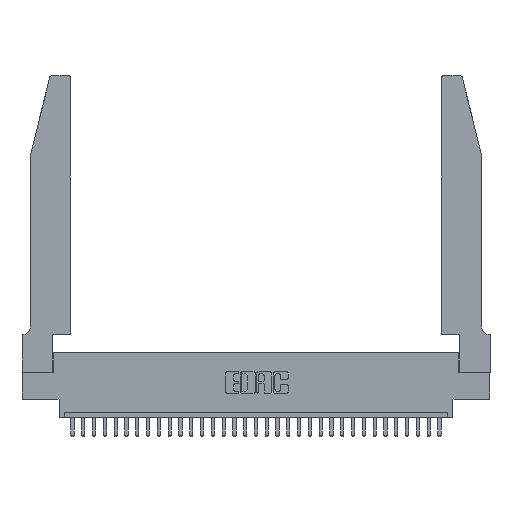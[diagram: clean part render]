
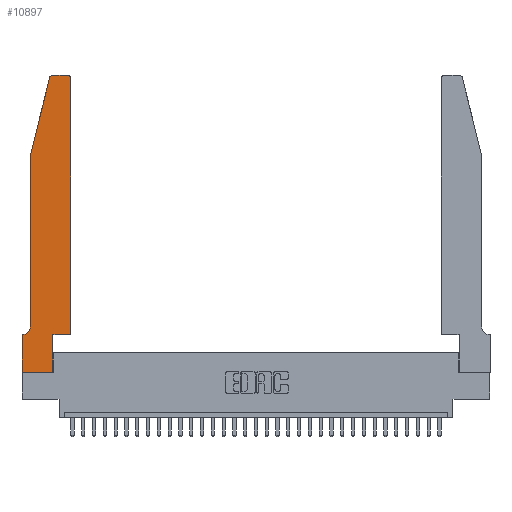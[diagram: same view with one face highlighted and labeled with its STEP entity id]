
A CAD part, top view. The second image highlights one B-rep face of the part: STEP entity #10897.
In plain terms, the highlighted planar face has unit normal (0, 0, 1).
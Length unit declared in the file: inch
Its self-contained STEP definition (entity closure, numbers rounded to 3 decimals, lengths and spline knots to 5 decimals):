
#288 = EDGE_CURVE ( 'NONE', #25515, #9720, #11505, .T. ) ;
#337 = CARTESIAN_POINT ( 'NONE',  ( 0.0755, 0.35, 0.37 ) ) ;
#338 = AXIS2_PLACEMENT_3D ( 'NONE', #15312, #20084, #5442 ) ;
#842 = CARTESIAN_POINT ( 'NONE',  ( 0.4505, 0.35, 0.37 ) ) ;
#1095 = CIRCLE ( 'NONE', #338, 0.07 ) ;
#1350 = LINE ( 'NONE', #337, #17381 ) ;
#1978 = DIRECTION ( 'NONE',  ( 1., 0., 0. ) ) ;
#2261 = CARTESIAN_POINT ( 'NONE',  ( 0., 0., 0.37 ) ) ;
#2297 = VECTOR ( 'NONE', #2922, 39.37008 ) ;
#2430 = LINE ( 'NONE', #842, #27750 ) ;
#2620 = AXIS2_PLACEMENT_3D ( 'NONE', #29353, #22128, #1978 ) ;
#2665 = DIRECTION ( 'NONE',  ( 1., 0., 0. ) ) ;
#2747 = EDGE_CURVE ( 'NONE', #4205, #11671, #27266, .T. ) ;
#2922 = DIRECTION ( 'NONE',  ( 0., -1., 0. ) ) ;
#2990 = EDGE_CURVE ( 'NONE', #8826, #29531, #31947, .T. ) ;
#3583 = DIRECTION ( 'NONE',  ( 0., 0., 1. ) ) ;
#3702 = LINE ( 'NONE', #25775, #23159 ) ;
#4205 = VERTEX_POINT ( 'NONE', #22556 ) ;
#4235 = ORIENTED_EDGE ( 'NONE', *, *, #18736, .T. ) ;
#4410 = ORIENTED_EDGE ( 'NONE', *, *, #7849, .T. ) ;
#4670 = CARTESIAN_POINT ( 'NONE',  ( 0.25487, 2.72718, 0.37 ) ) ;
#5312 = EDGE_CURVE ( 'NONE', #27766, #30841, #1350, .T. ) ;
#5442 = DIRECTION ( 'NONE',  ( -1., 0., 0. ) ) ;
#6222 = CARTESIAN_POINT ( 'NONE',  ( 0., 0., 0.37 ) ) ;
#6367 = EDGE_CURVE ( 'NONE', #29531, #7281, #2430, .T. ) ;
#6573 = CARTESIAN_POINT ( 'NONE',  ( 0.2865, 0.35, 0.37 ) ) ;
#6675 = DIRECTION ( 'NONE',  ( 0., 0., 1. ) ) ;
#7056 = VERTEX_POINT ( 'NONE', #22757 ) ;
#7281 = VERTEX_POINT ( 'NONE', #18565 ) ;
#7483 = VERTEX_POINT ( 'NONE', #4670 ) ;
#7849 = EDGE_CURVE ( 'NONE', #19479, #7056, #23005, .T. ) ;
#8826 = VERTEX_POINT ( 'NONE', #16630 ) ;
#8914 = EDGE_CURVE ( 'NONE', #7281, #25515, #17778, .T. ) ;
#9720 = VERTEX_POINT ( 'NONE', #16822 ) ;
#9958 = DIRECTION ( 'NONE',  ( -1., 0., 0. ) ) ;
#10822 = VECTOR ( 'NONE', #31478, 39.37008 ) ;
#10856 = CARTESIAN_POINT ( 'NONE',  ( 0.4205, 2.75, 0.37 ) ) ;
#10863 = DIRECTION ( 'NONE',  ( -0.239, -0.971, 0. ) ) ;
#10866 = ORIENTED_EDGE ( 'NONE', *, *, #20141, .T. ) ;
#10897 = ADVANCED_FACE ( 'NONE', ( #13824 ), #30630, .T. ) ;
#11071 = CARTESIAN_POINT ( 'NONE',  ( 0.0755, 0.42, 0.37 ) ) ;
#11104 = ORIENTED_EDGE ( 'NONE', *, *, #5312, .T. ) ;
#11374 = VECTOR ( 'NONE', #19668, 39.37008 ) ;
#11505 = LINE ( 'NONE', #16515, #17759 ) ;
#11671 = VERTEX_POINT ( 'NONE', #11071 ) ;
#11801 = EDGE_CURVE ( 'NONE', #7056, #8826, #19163, .T. ) ;
#11995 = EDGE_LOOP ( 'NONE', ( #30295, #13673, #10866, #31171, #4235, #11104, #22237, #4410, #24496, #26768, #27505, #30880 ) ) ;
#12178 = VECTOR ( 'NONE', #2665, 39.37008 ) ;
#13673 = ORIENTED_EDGE ( 'NONE', *, *, #29456, .T. ) ;
#13824 = FACE_OUTER_BOUND ( 'NONE', #11995, .T. ) ;
#13896 = EDGE_CURVE ( 'NONE', #30841, #19479, #30276, .T. ) ;
#14368 = CARTESIAN_POINT ( 'NONE',  ( 0.4205, 2.72, 0.37 ) ) ;
#14423 = CARTESIAN_POINT ( 'NONE',  ( 0.4505, 0.35, 0.37 ) ) ;
#14722 = CARTESIAN_POINT ( 'NONE',  ( 0., 0.35, 0.37 ) ) ;
#15312 = CARTESIAN_POINT ( 'NONE',  ( 0.0055, 0.42, 0.37 ) ) ;
#16475 = CARTESIAN_POINT ( 'NONE',  ( 0., 0., 0.37 ) ) ;
#16476 = DIRECTION ( 'NONE',  ( 1., 0., 0. ) ) ;
#16515 = CARTESIAN_POINT ( 'NONE',  ( 0.2605, 2.75, 0.37 ) ) ;
#16623 = DIRECTION ( 'NONE',  ( -1., 0., 0. ) ) ;
#16630 = CARTESIAN_POINT ( 'NONE',  ( 0.2865, 0.35, 0.37 ) ) ;
#16822 = CARTESIAN_POINT ( 'NONE',  ( 0.284, 2.75, 0.37 ) ) ;
#17381 = VECTOR ( 'NONE', #9958, 39.37008 ) ;
#17759 = VECTOR ( 'NONE', #16623, 39.37008 ) ;
#17778 = CIRCLE ( 'NONE', #24903, 0.03 ) ;
#17913 = CARTESIAN_POINT ( 'NONE',  ( 0.4505, 0.35, 0.37 ) ) ;
#18439 = DIRECTION ( 'NONE',  ( 0., 1., 0. ) ) ;
#18565 = CARTESIAN_POINT ( 'NONE',  ( 0.4505, 2.72, 0.37 ) ) ;
#18736 = EDGE_CURVE ( 'NONE', #11671, #27766, #1095, .T. ) ;
#19163 = LINE ( 'NONE', #6573, #11374 ) ;
#19479 = VERTEX_POINT ( 'NONE', #6222 ) ;
#19668 = DIRECTION ( 'NONE',  ( 0., 1., 0. ) ) ;
#20084 = DIRECTION ( 'NONE',  ( 0., 0., -1. ) ) ;
#20141 = EDGE_CURVE ( 'NONE', #7483, #4205, #3702, .T. ) ;
#22128 = DIRECTION ( 'NONE',  ( 0., 0., 1. ) ) ;
#22237 = ORIENTED_EDGE ( 'NONE', *, *, #13896, .T. ) ;
#22556 = CARTESIAN_POINT ( 'NONE',  ( 0.0755, 2., 0.37 ) ) ;
#22757 = CARTESIAN_POINT ( 'NONE',  ( 0.2865, 0., 0.37 ) ) ;
#23005 = LINE ( 'NONE', #2261, #12178 ) ;
#23159 = VECTOR ( 'NONE', #10863, 39.37008 ) ;
#23515 = DIRECTION ( 'NONE',  ( 1., 0., 0. ) ) ;
#24496 = ORIENTED_EDGE ( 'NONE', *, *, #11801, .T. ) ;
#24555 = CIRCLE ( 'NONE', #2620, 0.03 ) ;
#24903 = AXIS2_PLACEMENT_3D ( 'NONE', #14368, #6675, #29225 ) ;
#25269 = VECTOR ( 'NONE', #16476, 39.37008 ) ;
#25280 = CARTESIAN_POINT ( 'NONE',  ( 0.0755, 2., 0.37 ) ) ;
#25515 = VERTEX_POINT ( 'NONE', #10856 ) ;
#25775 = CARTESIAN_POINT ( 'NONE',  ( 0.0755, 2., 0.37 ) ) ;
#26768 = ORIENTED_EDGE ( 'NONE', *, *, #2990, .T. ) ;
#27266 = LINE ( 'NONE', #25280, #2297 ) ;
#27505 = ORIENTED_EDGE ( 'NONE', *, *, #6367, .T. ) ;
#27750 = VECTOR ( 'NONE', #18439, 39.37008 ) ;
#27766 = VERTEX_POINT ( 'NONE', #29451 ) ;
#29225 = DIRECTION ( 'NONE',  ( 1., 0., 0. ) ) ;
#29353 = CARTESIAN_POINT ( 'NONE',  ( 0.284, 2.72, 0.37 ) ) ;
#29358 = AXIS2_PLACEMENT_3D ( 'NONE', #30952, #3583, #23515 ) ;
#29451 = CARTESIAN_POINT ( 'NONE',  ( 0.0055, 0.35, 0.37 ) ) ;
#29456 = EDGE_CURVE ( 'NONE', #9720, #7483, #24555, .T. ) ;
#29531 = VERTEX_POINT ( 'NONE', #17913 ) ;
#30276 = LINE ( 'NONE', #16475, #10822 ) ;
#30295 = ORIENTED_EDGE ( 'NONE', *, *, #288, .T. ) ;
#30630 = PLANE ( 'NONE',  #29358 ) ;
#30841 = VERTEX_POINT ( 'NONE', #14722 ) ;
#30880 = ORIENTED_EDGE ( 'NONE', *, *, #8914, .T. ) ;
#30952 = CARTESIAN_POINT ( 'NONE',  ( 0., 0.35, 0.37 ) ) ;
#31171 = ORIENTED_EDGE ( 'NONE', *, *, #2747, .T. ) ;
#31478 = DIRECTION ( 'NONE',  ( 0., -1., 0. ) ) ;
#31947 = LINE ( 'NONE', #14423, #25269 ) ;
